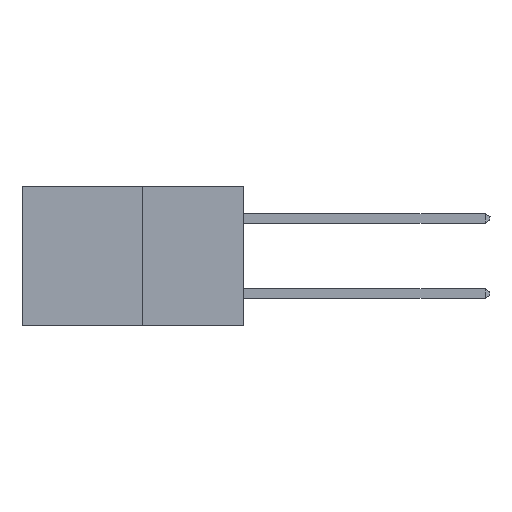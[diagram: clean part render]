
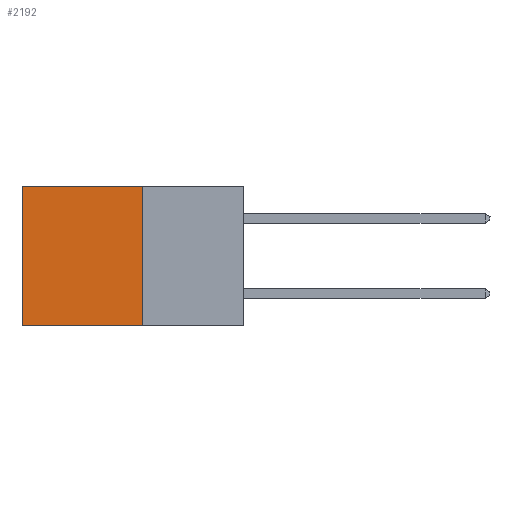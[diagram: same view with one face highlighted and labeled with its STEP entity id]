
A CAD part, left-side view. The second image highlights one B-rep face of the part: STEP entity #2192.
In plain terms, the highlighted planar face has unit normal (-1, 0, 0).
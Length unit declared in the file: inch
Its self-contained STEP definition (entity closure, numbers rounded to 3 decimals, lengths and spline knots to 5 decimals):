
#105 = ORIENTED_EDGE ( 'NONE', *, *, #2828, .F. ) ;
#190 = LINE ( 'NONE', #7669, #5514 ) ;
#240 = ORIENTED_EDGE ( 'NONE', *, *, #5093, .F. ) ;
#503 = DIRECTION ( 'NONE',  ( 0., 1., 0. ) ) ;
#721 = CARTESIAN_POINT ( 'NONE',  ( 0.277, 0.27, 0. ) ) ;
#810 = DIRECTION ( 'NONE',  ( 0., 0., -1. ) ) ;
#1327 = ORIENTED_EDGE ( 'NONE', *, *, #8281, .T. ) ;
#1556 = AXIS2_PLACEMENT_3D ( 'NONE', #6785, #6399, #6069 ) ;
#2192 = ADVANCED_FACE ( 'NONE', ( #5170 ), #8378, .F. ) ;
#2619 = VERTEX_POINT ( 'NONE', #3241 ) ;
#2828 = EDGE_CURVE ( 'NONE', #7167, #6345, #7497, .T. ) ;
#3038 = VECTOR ( 'NONE', #4245, 39.37008 ) ;
#3056 = CARTESIAN_POINT ( 'NONE',  ( 0.277, 0.59, 0. ) ) ;
#3241 = CARTESIAN_POINT ( 'NONE',  ( 0.277, 0.59, -0.37 ) ) ;
#3670 = EDGE_LOOP ( 'NONE', ( #1327, #240, #105, #7132 ) ) ;
#3882 = VECTOR ( 'NONE', #810, 39.37008 ) ;
#4245 = DIRECTION ( 'NONE',  ( 0., 0., -1. ) ) ;
#4832 = VECTOR ( 'NONE', #503, 39.37008 ) ;
#4852 = LINE ( 'NONE', #6777, #3038 ) ;
#4948 = EDGE_CURVE ( 'NONE', #7167, #5590, #5001, .T. ) ;
#5001 = LINE ( 'NONE', #721, #4832 ) ;
#5093 = EDGE_CURVE ( 'NONE', #6345, #2619, #190, .T. ) ;
#5170 = FACE_OUTER_BOUND ( 'NONE', #3670, .T. ) ;
#5181 = CARTESIAN_POINT ( 'NONE',  ( 0.277, 0.27, 0. ) ) ;
#5514 = VECTOR ( 'NONE', #7726, 39.37008 ) ;
#5590 = VERTEX_POINT ( 'NONE', #3056 ) ;
#6049 = CARTESIAN_POINT ( 'NONE',  ( 0.277, 0.27, -0.37 ) ) ;
#6069 = DIRECTION ( 'NONE',  ( 0., 0., -1. ) ) ;
#6345 = VERTEX_POINT ( 'NONE', #7540 ) ;
#6399 = DIRECTION ( 'NONE',  ( 1., 0., 0. ) ) ;
#6777 = CARTESIAN_POINT ( 'NONE',  ( 0.277, 0.59, -0.37 ) ) ;
#6785 = CARTESIAN_POINT ( 'NONE',  ( 0.277, 0.27, -0.37 ) ) ;
#7132 = ORIENTED_EDGE ( 'NONE', *, *, #4948, .T. ) ;
#7167 = VERTEX_POINT ( 'NONE', #5181 ) ;
#7497 = LINE ( 'NONE', #6049, #3882 ) ;
#7540 = CARTESIAN_POINT ( 'NONE',  ( 0.277, 0.27, -0.37 ) ) ;
#7669 = CARTESIAN_POINT ( 'NONE',  ( 0.277, 0.27, -0.37 ) ) ;
#7726 = DIRECTION ( 'NONE',  ( 0., 1., 0. ) ) ;
#8281 = EDGE_CURVE ( 'NONE', #5590, #2619, #4852, .T. ) ;
#8378 = PLANE ( 'NONE',  #1556 ) ;
